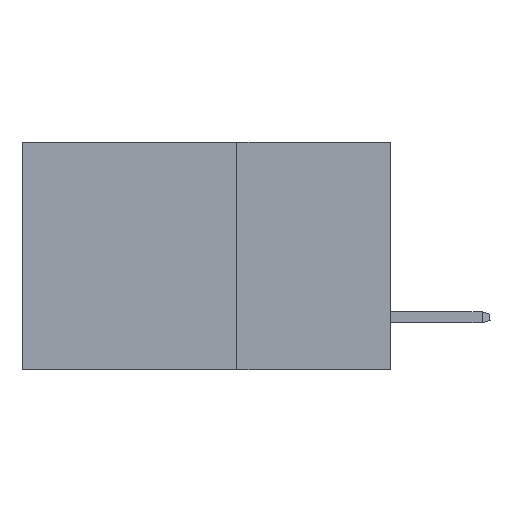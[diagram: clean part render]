
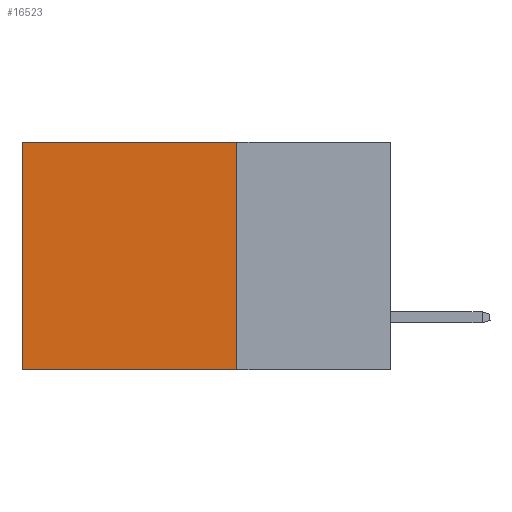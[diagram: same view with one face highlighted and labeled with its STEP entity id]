
A CAD part, left-side view. The second image highlights one B-rep face of the part: STEP entity #16523.
In plain terms, the highlighted planar face has unit normal (-1, 0, 0).
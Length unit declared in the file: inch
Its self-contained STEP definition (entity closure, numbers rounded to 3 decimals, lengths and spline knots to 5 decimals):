
#33 = VERTEX_POINT ( 'NONE', #4308 ) ;
#750 = CARTESIAN_POINT ( 'NONE',  ( 0.2875, 0.6, 0. ) ) ;
#1333 = ORIENTED_EDGE ( 'NONE', *, *, #19976, .T. ) ;
#1614 = EDGE_LOOP ( 'NONE', ( #1333, #15702, #21150, #5134 ) ) ;
#4308 = CARTESIAN_POINT ( 'NONE',  ( 0.2875, 0.25, 0. ) ) ;
#5003 = LINE ( 'NONE', #750, #6489 ) ;
#5134 = ORIENTED_EDGE ( 'NONE', *, *, #29201, .T. ) ;
#5403 = DIRECTION ( 'NONE',  ( 0., 1., 0. ) ) ;
#6489 = VECTOR ( 'NONE', #27488, 39.37008 ) ;
#7283 = VECTOR ( 'NONE', #5403, 39.37008 ) ;
#7725 = DIRECTION ( 'NONE',  ( 1., 0., 0. ) ) ;
#7831 = CARTESIAN_POINT ( 'NONE',  ( 0.2875, 0.25, 0. ) ) ;
#10747 = LINE ( 'NONE', #7831, #24682 ) ;
#10995 = AXIS2_PLACEMENT_3D ( 'NONE', #24093, #7725, #19228 ) ;
#10999 = CARTESIAN_POINT ( 'NONE',  ( 0.2875, 0.6, 0. ) ) ;
#11548 = FACE_OUTER_BOUND ( 'NONE', #1614, .T. ) ;
#11679 = DIRECTION ( 'NONE',  ( 0., 1., 0. ) ) ;
#13466 = CARTESIAN_POINT ( 'NONE',  ( 0.2875, 0.25, -0.37 ) ) ;
#14264 = LINE ( 'NONE', #16664, #7283 ) ;
#15702 = ORIENTED_EDGE ( 'NONE', *, *, #30194, .F. ) ;
#16523 = ADVANCED_FACE ( 'NONE', ( #11548 ), #26459, .F. ) ;
#16664 = CARTESIAN_POINT ( 'NONE',  ( 0.2875, 0.25, 0. ) ) ;
#18263 = VECTOR ( 'NONE', #11679, 39.37008 ) ;
#18966 = LINE ( 'NONE', #13466, #18263 ) ;
#19228 = DIRECTION ( 'NONE',  ( 0., 0., -1. ) ) ;
#19976 = EDGE_CURVE ( 'NONE', #21338, #24871, #5003, .T. ) ;
#20532 = VERTEX_POINT ( 'NONE', #23374 ) ;
#21150 = ORIENTED_EDGE ( 'NONE', *, *, #21898, .F. ) ;
#21338 = VERTEX_POINT ( 'NONE', #10999 ) ;
#21898 = EDGE_CURVE ( 'NONE', #33, #20532, #10747, .T. ) ;
#23166 = CARTESIAN_POINT ( 'NONE',  ( 0.2875, 0.6, -0.37 ) ) ;
#23374 = CARTESIAN_POINT ( 'NONE',  ( 0.2875, 0.25, -0.37 ) ) ;
#24093 = CARTESIAN_POINT ( 'NONE',  ( 0.2875, 0.25, 0. ) ) ;
#24682 = VECTOR ( 'NONE', #26128, 39.37008 ) ;
#24871 = VERTEX_POINT ( 'NONE', #23166 ) ;
#26128 = DIRECTION ( 'NONE',  ( 0., 0., -1. ) ) ;
#26459 = PLANE ( 'NONE',  #10995 ) ;
#27488 = DIRECTION ( 'NONE',  ( 0., 0., -1. ) ) ;
#29201 = EDGE_CURVE ( 'NONE', #33, #21338, #14264, .T. ) ;
#30194 = EDGE_CURVE ( 'NONE', #20532, #24871, #18966, .T. ) ;
